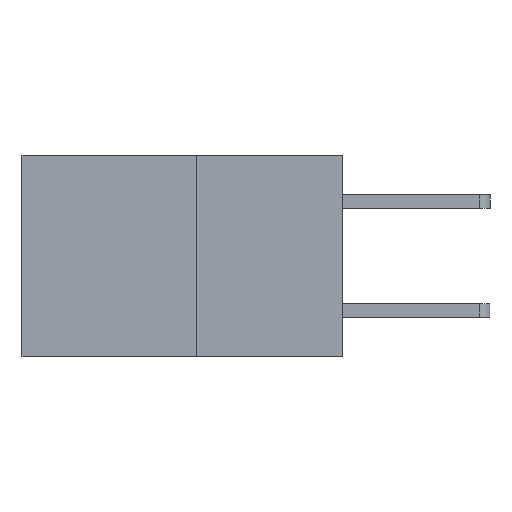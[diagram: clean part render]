
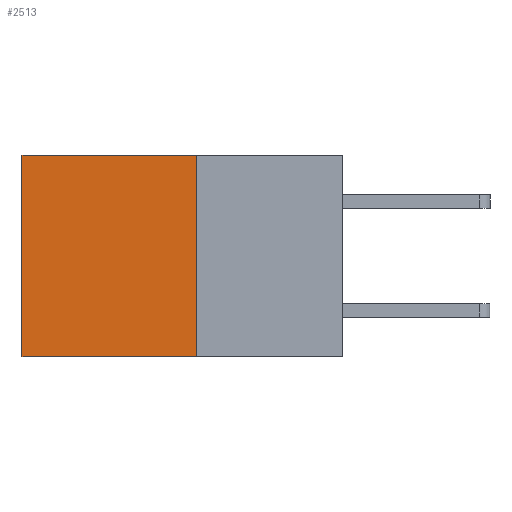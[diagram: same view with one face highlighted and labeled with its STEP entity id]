
A CAD part, left-side view. The second image highlights one B-rep face of the part: STEP entity #2513.
In plain terms, the highlighted planar face has unit normal (-1, 0, 0).
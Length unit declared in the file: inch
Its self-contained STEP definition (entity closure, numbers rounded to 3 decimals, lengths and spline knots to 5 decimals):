
#37 = VECTOR ( 'NONE', #6910, 39.37008 ) ;
#50 = VERTEX_POINT ( 'NONE', #1988 ) ;
#204 = PLANE ( 'NONE',  #2717 ) ;
#281 = DIRECTION ( 'NONE',  ( 0., 0., -1. ) ) ;
#732 = CARTESIAN_POINT ( 'NONE',  ( 0.277, 0.59, 0. ) ) ;
#1269 = VECTOR ( 'NONE', #8223, 39.37008 ) ;
#1556 = CARTESIAN_POINT ( 'NONE',  ( 0.277, 0.27, -0.37 ) ) ;
#1646 = CARTESIAN_POINT ( 'NONE',  ( 0.277, 0.27, -0.37 ) ) ;
#1732 = LINE ( 'NONE', #2379, #1971 ) ;
#1793 = ORIENTED_EDGE ( 'NONE', *, *, #6795, .F. ) ;
#1971 = VECTOR ( 'NONE', #5081, 39.37008 ) ;
#1988 = CARTESIAN_POINT ( 'NONE',  ( 0.277, 0.59, -0.37 ) ) ;
#2169 = LINE ( 'NONE', #2185, #37 ) ;
#2185 = CARTESIAN_POINT ( 'NONE',  ( 0.277, 0.27, -0.37 ) ) ;
#2315 = ORIENTED_EDGE ( 'NONE', *, *, #3362, .T. ) ;
#2379 = CARTESIAN_POINT ( 'NONE',  ( 0.277, 0.59, -0.37 ) ) ;
#2428 = CARTESIAN_POINT ( 'NONE',  ( 0.277, 0.27, 0. ) ) ;
#2506 = CARTESIAN_POINT ( 'NONE',  ( 0.277, 0.27, -0.37 ) ) ;
#2513 = ADVANCED_FACE ( 'NONE', ( #7134 ), #204, .F. ) ;
#2533 = ORIENTED_EDGE ( 'NONE', *, *, #4850, .T. ) ;
#2717 = AXIS2_PLACEMENT_3D ( 'NONE', #2506, #6930, #281 ) ;
#2732 = ORIENTED_EDGE ( 'NONE', *, *, #4237, .F. ) ;
#3362 = EDGE_CURVE ( 'NONE', #6770, #50, #1732, .T. ) ;
#3594 = VECTOR ( 'NONE', #8331, 39.37008 ) ;
#4237 = EDGE_CURVE ( 'NONE', #4839, #7652, #2169, .T. ) ;
#4839 = VERTEX_POINT ( 'NONE', #2428 ) ;
#4850 = EDGE_CURVE ( 'NONE', #4839, #6770, #8351, .T. ) ;
#5081 = DIRECTION ( 'NONE',  ( 0., 0., -1. ) ) ;
#6716 = EDGE_LOOP ( 'NONE', ( #2315, #1793, #2732, #2533 ) ) ;
#6770 = VERTEX_POINT ( 'NONE', #732 ) ;
#6795 = EDGE_CURVE ( 'NONE', #7652, #50, #8400, .T. ) ;
#6910 = DIRECTION ( 'NONE',  ( 0., 0., -1. ) ) ;
#6930 = DIRECTION ( 'NONE',  ( 1., 0., 0. ) ) ;
#7134 = FACE_OUTER_BOUND ( 'NONE', #6716, .T. ) ;
#7652 = VERTEX_POINT ( 'NONE', #1646 ) ;
#7676 = CARTESIAN_POINT ( 'NONE',  ( 0.277, 0.27, 0. ) ) ;
#8223 = DIRECTION ( 'NONE',  ( 0., 1., 0. ) ) ;
#8331 = DIRECTION ( 'NONE',  ( 0., 1., 0. ) ) ;
#8351 = LINE ( 'NONE', #7676, #3594 ) ;
#8400 = LINE ( 'NONE', #1556, #1269 ) ;
